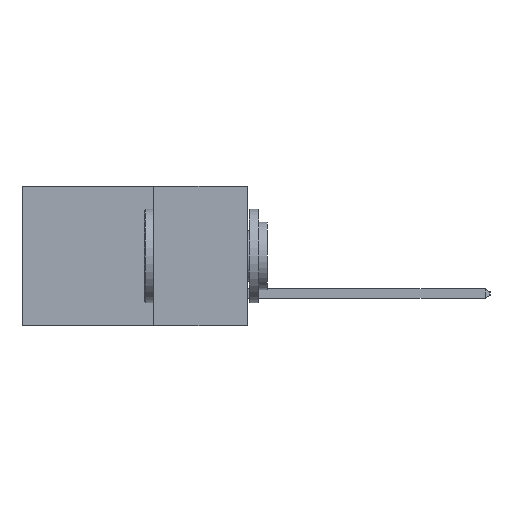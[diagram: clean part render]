
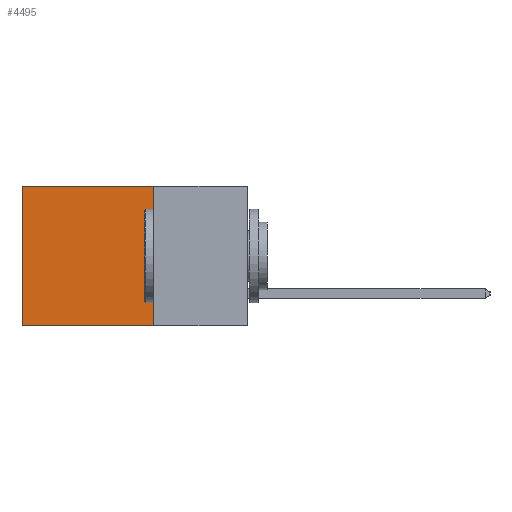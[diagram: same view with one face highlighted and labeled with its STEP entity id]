
A CAD part, left-side view. The second image highlights one B-rep face of the part: STEP entity #4495.
In plain terms, the highlighted planar face has unit normal (-1, 0, 0).
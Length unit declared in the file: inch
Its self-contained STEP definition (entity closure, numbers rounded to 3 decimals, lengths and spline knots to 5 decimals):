
#397 = CARTESIAN_POINT ( 'NONE',  ( 0.298, 0.6, 0. ) ) ;
#430 = VERTEX_POINT ( 'NONE', #8962 ) ;
#861 = ORIENTED_EDGE ( 'NONE', *, *, #2790, .F. ) ;
#1947 = CARTESIAN_POINT ( 'NONE',  ( 0.298, 0.6, 0. ) ) ;
#2453 = PLANE ( 'NONE',  #8690 ) ;
#2485 = LINE ( 'NONE', #5359, #6764 ) ;
#2591 = FACE_OUTER_BOUND ( 'NONE', #6039, .T. ) ;
#2790 = EDGE_CURVE ( 'NONE', #10320, #5155, #2485, .T. ) ;
#3125 = LINE ( 'NONE', #6394, #7207 ) ;
#4440 = EDGE_CURVE ( 'NONE', #10320, #6310, #3125, .T. ) ;
#4491 = DIRECTION ( 'NONE',  ( 0., 0., -1. ) ) ;
#4495 = ADVANCED_FACE ( 'NONE', ( #2591 ), #2453, .F. ) ;
#4529 = DIRECTION ( 'NONE',  ( 1., 0., 0. ) ) ;
#4717 = ORIENTED_EDGE ( 'NONE', *, *, #7329, .F. ) ;
#5155 = VERTEX_POINT ( 'NONE', #6683 ) ;
#5359 = CARTESIAN_POINT ( 'NONE',  ( 0.298, 0.25, 0. ) ) ;
#5363 = DIRECTION ( 'NONE',  ( 0., 0., -1. ) ) ;
#5565 = ORIENTED_EDGE ( 'NONE', *, *, #4440, .T. ) ;
#5922 = VECTOR ( 'NONE', #9560, 39.37008 ) ;
#6039 = EDGE_LOOP ( 'NONE', ( #10135, #4717, #861, #5565 ) ) ;
#6310 = VERTEX_POINT ( 'NONE', #1947 ) ;
#6348 = DIRECTION ( 'NONE',  ( 0., 0., -1. ) ) ;
#6394 = CARTESIAN_POINT ( 'NONE',  ( 0.298, 0.25, 0. ) ) ;
#6683 = CARTESIAN_POINT ( 'NONE',  ( 0.298, 0.25, -0.37 ) ) ;
#6764 = VECTOR ( 'NONE', #5363, 39.37008 ) ;
#7063 = LINE ( 'NONE', #397, #9243 ) ;
#7207 = VECTOR ( 'NONE', #9694, 39.37008 ) ;
#7329 = EDGE_CURVE ( 'NONE', #5155, #430, #9922, .T. ) ;
#8499 = CARTESIAN_POINT ( 'NONE',  ( 0.298, 0.25, 0. ) ) ;
#8614 = EDGE_CURVE ( 'NONE', #6310, #430, #7063, .T. ) ;
#8690 = AXIS2_PLACEMENT_3D ( 'NONE', #9727, #4529, #4491 ) ;
#8962 = CARTESIAN_POINT ( 'NONE',  ( 0.298, 0.6, -0.37 ) ) ;
#9210 = CARTESIAN_POINT ( 'NONE',  ( 0.298, 0.25, -0.37 ) ) ;
#9243 = VECTOR ( 'NONE', #6348, 39.37008 ) ;
#9560 = DIRECTION ( 'NONE',  ( 0., 1., 0. ) ) ;
#9694 = DIRECTION ( 'NONE',  ( 0., 1., 0. ) ) ;
#9727 = CARTESIAN_POINT ( 'NONE',  ( 0.298, 0.25, 0. ) ) ;
#9922 = LINE ( 'NONE', #9210, #5922 ) ;
#10135 = ORIENTED_EDGE ( 'NONE', *, *, #8614, .T. ) ;
#10320 = VERTEX_POINT ( 'NONE', #8499 ) ;
